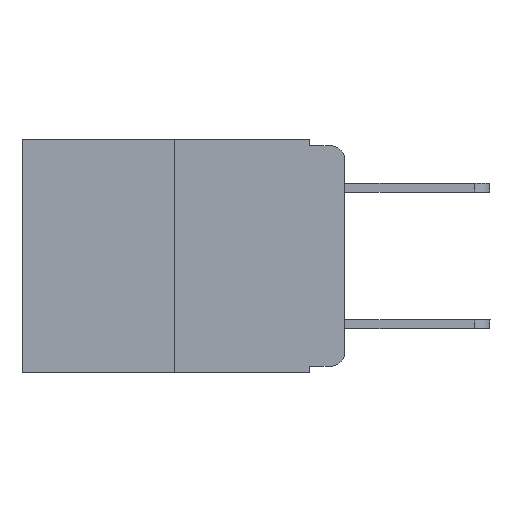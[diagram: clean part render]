
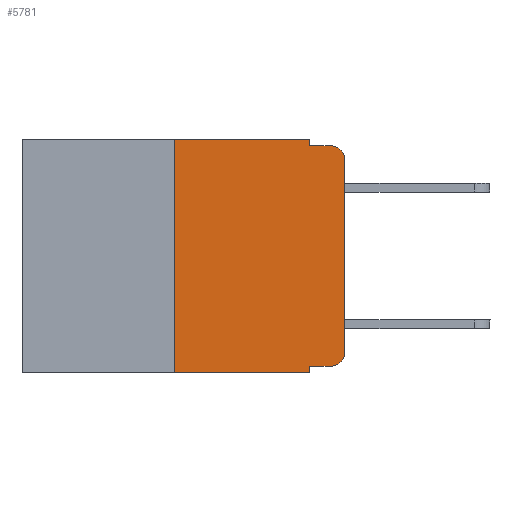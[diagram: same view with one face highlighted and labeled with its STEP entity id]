
A CAD part, left-side view. The second image highlights one B-rep face of the part: STEP entity #5781.
In plain terms, the highlighted planar face has unit normal (-1, 0, 0).
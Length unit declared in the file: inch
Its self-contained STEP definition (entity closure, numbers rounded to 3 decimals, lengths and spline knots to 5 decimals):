
#765 = CARTESIAN_POINT ( 'NONE',  ( 0., 0., -0.313 ) ) ;
#897 = DIRECTION ( 'NONE',  ( 0., 0., -1. ) ) ;
#996 = ORIENTED_EDGE ( 'NONE', *, *, #12657, .T. ) ;
#1147 = EDGE_CURVE ( 'NONE', #12033, #11844, #1229, .T. ) ;
#1229 = LINE ( 'NONE', #2925, #5135 ) ;
#1257 = ORIENTED_EDGE ( 'NONE', *, *, #2964, .F. ) ;
#1510 = VERTEX_POINT ( 'NONE', #8932 ) ;
#1663 = ORIENTED_EDGE ( 'NONE', *, *, #11835, .T. ) ;
#1747 = DIRECTION ( 'NONE',  ( 0., 0., -1. ) ) ;
#1780 = VECTOR ( 'NONE', #9898, 39.37008 ) ;
#1869 = VERTEX_POINT ( 'NONE', #2849 ) ;
#2046 = AXIS2_PLACEMENT_3D ( 'NONE', #10644, #13305, #5522 ) ;
#2084 = LINE ( 'NONE', #4301, #15901 ) ;
#2381 = ORIENTED_EDGE ( 'NONE', *, *, #15115, .T. ) ;
#2472 = VERTEX_POINT ( 'NONE', #765 ) ;
#2548 = EDGE_CURVE ( 'NONE', #3613, #12033, #12722, .T. ) ;
#2849 = CARTESIAN_POINT ( 'NONE',  ( 0., 0.051, -0.343 ) ) ;
#2925 = CARTESIAN_POINT ( 'NONE',  ( 0., 0.051, 0. ) ) ;
#2964 = EDGE_CURVE ( 'NONE', #1510, #3613, #16246, .T. ) ;
#3228 = DIRECTION ( 'NONE',  ( 0., -1., 0. ) ) ;
#3613 = VERTEX_POINT ( 'NONE', #13132 ) ;
#3675 = VECTOR ( 'NONE', #1747, 39.37008 ) ;
#3851 = CARTESIAN_POINT ( 'NONE',  ( 0., 0.051, -0.333 ) ) ;
#3898 = CARTESIAN_POINT ( 'NONE',  ( 0., 0.02, -0.313 ) ) ;
#3968 = DIRECTION ( 'NONE',  ( 0., 0., -1. ) ) ;
#4003 = AXIS2_PLACEMENT_3D ( 'NONE', #3898, #13334, #897 ) ;
#4301 = CARTESIAN_POINT ( 'NONE',  ( 0., 0.473, -0.343 ) ) ;
#4348 = CARTESIAN_POINT ( 'NONE',  ( 0., 0.051, -0.01 ) ) ;
#5135 = VECTOR ( 'NONE', #16066, 39.37008 ) ;
#5334 = ORIENTED_EDGE ( 'NONE', *, *, #7198, .T. ) ;
#5522 = DIRECTION ( 'NONE',  ( 0., 0., -1. ) ) ;
#5781 = ADVANCED_FACE ( 'NONE', ( #8262 ), #14589, .F. ) ;
#6457 = CARTESIAN_POINT ( 'NONE',  ( 0., 0.02, -0.01 ) ) ;
#6920 = DIRECTION ( 'NONE',  ( 0., -1., 0. ) ) ;
#7044 = ORIENTED_EDGE ( 'NONE', *, *, #1147, .F. ) ;
#7198 = EDGE_CURVE ( 'NONE', #1510, #1869, #2084, .T. ) ;
#7726 = EDGE_CURVE ( 'NONE', #11844, #14806, #13192, .T. ) ;
#8020 = VECTOR ( 'NONE', #6920, 39.37008 ) ;
#8262 = FACE_OUTER_BOUND ( 'NONE', #10102, .T. ) ;
#8348 = DIRECTION ( 'NONE',  ( 0., -1., 0. ) ) ;
#8907 = ORIENTED_EDGE ( 'NONE', *, *, #7726, .F. ) ;
#8932 = CARTESIAN_POINT ( 'NONE',  ( 0., 0.25, -0.343 ) ) ;
#9236 = EDGE_CURVE ( 'NONE', #9919, #1869, #10576, .T. ) ;
#9554 = CARTESIAN_POINT ( 'NONE',  ( 0., 0.051, -0.01 ) ) ;
#9692 = VERTEX_POINT ( 'NONE', #15150 ) ;
#9898 = DIRECTION ( 'NONE',  ( 0., 0., 1. ) ) ;
#9919 = VERTEX_POINT ( 'NONE', #3851 ) ;
#10024 = EDGE_CURVE ( 'NONE', #16094, #2472, #11426, .T. ) ;
#10102 = EDGE_LOOP ( 'NONE', ( #2381, #1663, #8907, #7044, #12099, #1257, #5334, #14752, #996, #12500 ) ) ;
#10357 = AXIS2_PLACEMENT_3D ( 'NONE', #15831, #12692, #3968 ) ;
#10491 = CARTESIAN_POINT ( 'NONE',  ( 0., 0.02, -0.333 ) ) ;
#10576 = LINE ( 'NONE', #12262, #3675 ) ;
#10644 = CARTESIAN_POINT ( 'NONE',  ( 0., 0.02, -0.03 ) ) ;
#11426 = CIRCLE ( 'NONE', #4003, 0.02 ) ;
#11835 = EDGE_CURVE ( 'NONE', #9692, #14806, #13234, .T. ) ;
#11844 = VERTEX_POINT ( 'NONE', #9554 ) ;
#11877 = VECTOR ( 'NONE', #16329, 39.37008 ) ;
#12033 = VERTEX_POINT ( 'NONE', #14043 ) ;
#12099 = ORIENTED_EDGE ( 'NONE', *, *, #2548, .F. ) ;
#12262 = CARTESIAN_POINT ( 'NONE',  ( 0., 0.051, 0. ) ) ;
#12276 = LINE ( 'NONE', #15154, #1780 ) ;
#12500 = ORIENTED_EDGE ( 'NONE', *, *, #10024, .T. ) ;
#12578 = LINE ( 'NONE', #13844, #15066 ) ;
#12657 = EDGE_CURVE ( 'NONE', #9919, #16094, #12578, .T. ) ;
#12692 = DIRECTION ( 'NONE',  ( 1., 0., 0. ) ) ;
#12722 = LINE ( 'NONE', #14986, #11877 ) ;
#13130 = VECTOR ( 'NONE', #16359, 39.37008 ) ;
#13132 = CARTESIAN_POINT ( 'NONE',  ( 0., 0.25, 0. ) ) ;
#13192 = LINE ( 'NONE', #4348, #8020 ) ;
#13234 = CIRCLE ( 'NONE', #2046, 0.02 ) ;
#13305 = DIRECTION ( 'NONE',  ( -1., 0., 0. ) ) ;
#13334 = DIRECTION ( 'NONE',  ( -1., 0., 0. ) ) ;
#13624 = CARTESIAN_POINT ( 'NONE',  ( 0., 0.25, 0. ) ) ;
#13844 = CARTESIAN_POINT ( 'NONE',  ( 0., 0.051, -0.333 ) ) ;
#14043 = CARTESIAN_POINT ( 'NONE',  ( 0., 0.051, 0. ) ) ;
#14589 = PLANE ( 'NONE',  #10357 ) ;
#14752 = ORIENTED_EDGE ( 'NONE', *, *, #9236, .F. ) ;
#14806 = VERTEX_POINT ( 'NONE', #6457 ) ;
#14986 = CARTESIAN_POINT ( 'NONE',  ( 0., 0.473, 0. ) ) ;
#15066 = VECTOR ( 'NONE', #8348, 39.37008 ) ;
#15115 = EDGE_CURVE ( 'NONE', #2472, #9692, #12276, .T. ) ;
#15150 = CARTESIAN_POINT ( 'NONE',  ( 0., 0., -0.03 ) ) ;
#15154 = CARTESIAN_POINT ( 'NONE',  ( 0., 0., 0. ) ) ;
#15831 = CARTESIAN_POINT ( 'NONE',  ( 0., 0.473, 0. ) ) ;
#15901 = VECTOR ( 'NONE', #3228, 39.37008 ) ;
#16066 = DIRECTION ( 'NONE',  ( 0., 0., -1. ) ) ;
#16094 = VERTEX_POINT ( 'NONE', #10491 ) ;
#16246 = LINE ( 'NONE', #13624, #13130 ) ;
#16329 = DIRECTION ( 'NONE',  ( 0., -1., 0. ) ) ;
#16359 = DIRECTION ( 'NONE',  ( 0., 0., 1. ) ) ;
